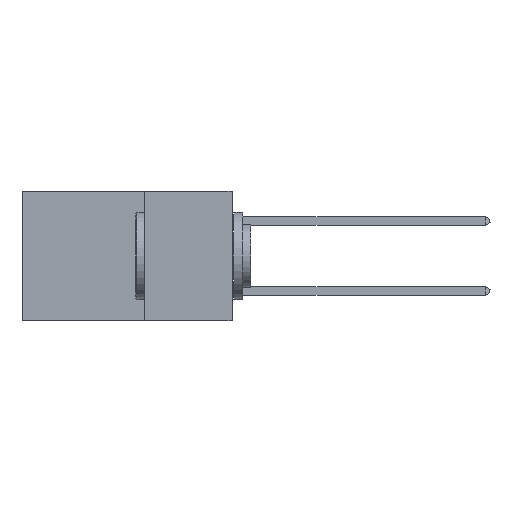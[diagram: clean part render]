
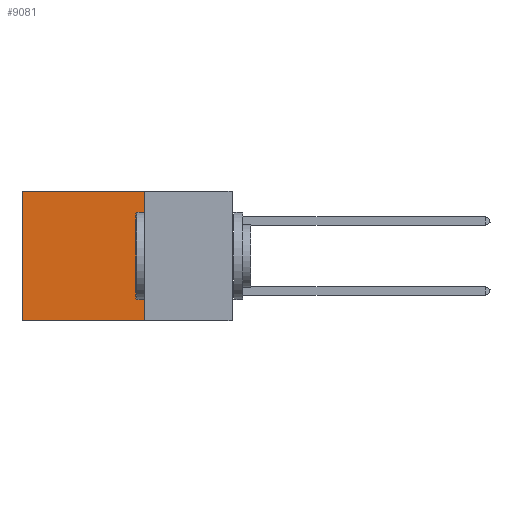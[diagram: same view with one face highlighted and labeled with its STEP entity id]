
A CAD part, left-side view. The second image highlights one B-rep face of the part: STEP entity #9081.
In plain terms, the highlighted planar face has unit normal (-1, 0, 0).
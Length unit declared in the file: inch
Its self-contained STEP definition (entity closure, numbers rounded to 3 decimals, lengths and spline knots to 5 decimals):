
#1927 = VERTEX_POINT ( 'NONE', #19848 ) ;
#2249 = ORIENTED_EDGE ( 'NONE', *, *, #29058, .F. ) ;
#3108 = VECTOR ( 'NONE', #21264, 39.37008 ) ;
#3591 = LINE ( 'NONE', #4871, #16109 ) ;
#3780 = VERTEX_POINT ( 'NONE', #4985 ) ;
#4871 = CARTESIAN_POINT ( 'NONE',  ( 0.2875, 0.25, 0. ) ) ;
#4985 = CARTESIAN_POINT ( 'NONE',  ( 0.2875, 0.6, 0. ) ) ;
#6201 = VECTOR ( 'NONE', #17350, 39.37008 ) ;
#7316 = EDGE_CURVE ( 'NONE', #1927, #23556, #3591, .T. ) ;
#7407 = PLANE ( 'NONE',  #27365 ) ;
#8372 = CARTESIAN_POINT ( 'NONE',  ( 0.2875, 0.25, -0.37 ) ) ;
#9081 = ADVANCED_FACE ( 'NONE', ( #28736 ), #7407, .F. ) ;
#9250 = EDGE_LOOP ( 'NONE', ( #20768, #2249, #26790, #27841 ) ) ;
#9455 = LINE ( 'NONE', #23491, #3108 ) ;
#9546 = DIRECTION ( 'NONE',  ( 0., 0., -1. ) ) ;
#10769 = DIRECTION ( 'NONE',  ( 0., 1., 0. ) ) ;
#10997 = CARTESIAN_POINT ( 'NONE',  ( 0.2875, 0.25, -0.37 ) ) ;
#12151 = DIRECTION ( 'NONE',  ( 0., 0., -1. ) ) ;
#13195 = LINE ( 'NONE', #28891, #6201 ) ;
#14658 = CARTESIAN_POINT ( 'NONE',  ( 0.2875, 0.6, -0.37 ) ) ;
#15983 = VECTOR ( 'NONE', #10769, 39.37008 ) ;
#16109 = VECTOR ( 'NONE', #9546, 39.37008 ) ;
#17350 = DIRECTION ( 'NONE',  ( 0., 0., -1. ) ) ;
#17503 = EDGE_CURVE ( 'NONE', #3780, #26348, #13195, .T. ) ;
#19184 = EDGE_CURVE ( 'NONE', #1927, #3780, #9455, .T. ) ;
#19848 = CARTESIAN_POINT ( 'NONE',  ( 0.2875, 0.25, 0. ) ) ;
#20768 = ORIENTED_EDGE ( 'NONE', *, *, #17503, .T. ) ;
#21264 = DIRECTION ( 'NONE',  ( 0., 1., 0. ) ) ;
#23491 = CARTESIAN_POINT ( 'NONE',  ( 0.2875, 0.25, 0. ) ) ;
#23556 = VERTEX_POINT ( 'NONE', #10997 ) ;
#23754 = CARTESIAN_POINT ( 'NONE',  ( 0.2875, 0.25, 0. ) ) ;
#26105 = DIRECTION ( 'NONE',  ( 1., 0., 0. ) ) ;
#26348 = VERTEX_POINT ( 'NONE', #14658 ) ;
#26790 = ORIENTED_EDGE ( 'NONE', *, *, #7316, .F. ) ;
#27365 = AXIS2_PLACEMENT_3D ( 'NONE', #23754, #26105, #12151 ) ;
#27841 = ORIENTED_EDGE ( 'NONE', *, *, #19184, .T. ) ;
#28322 = LINE ( 'NONE', #8372, #15983 ) ;
#28736 = FACE_OUTER_BOUND ( 'NONE', #9250, .T. ) ;
#28891 = CARTESIAN_POINT ( 'NONE',  ( 0.2875, 0.6, 0. ) ) ;
#29058 = EDGE_CURVE ( 'NONE', #23556, #26348, #28322, .T. ) ;
